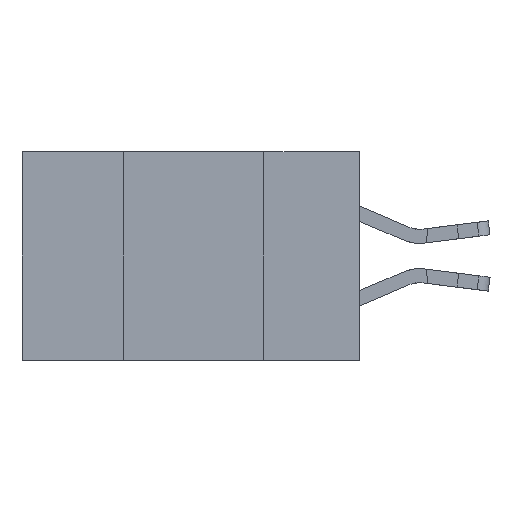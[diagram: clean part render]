
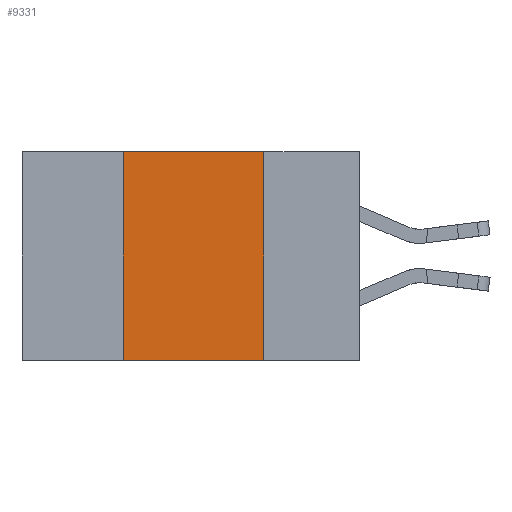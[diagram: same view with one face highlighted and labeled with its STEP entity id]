
A CAD part, left-side view. The second image highlights one B-rep face of the part: STEP entity #9331.
In plain terms, the highlighted planar face has unit normal (-1, 0, 0).
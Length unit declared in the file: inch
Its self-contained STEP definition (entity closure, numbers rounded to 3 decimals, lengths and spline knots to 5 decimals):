
#10 = LINE ( 'NONE', #21667, #20473 ) ;
#77 = ORIENTED_EDGE ( 'NONE', *, *, #8759, .F. ) ;
#528 = DIRECTION ( 'NONE',  ( 0., -1., 0. ) ) ;
#727 = VECTOR ( 'NONE', #10962, 39.37008 ) ;
#1062 = EDGE_CURVE ( 'NONE', #15115, #17865, #5064, .T. ) ;
#2873 = FACE_OUTER_BOUND ( 'NONE', #7332, .T. ) ;
#3365 = EDGE_CURVE ( 'NONE', #15115, #3771, #10, .T. ) ;
#3537 = LINE ( 'NONE', #15646, #3848 ) ;
#3771 = VERTEX_POINT ( 'NONE', #7977 ) ;
#3848 = VECTOR ( 'NONE', #25251, 39.37008 ) ;
#3983 = DIRECTION ( 'NONE',  ( 0., 0., 1. ) ) ;
#5064 = LINE ( 'NONE', #12418, #20917 ) ;
#7332 = EDGE_LOOP ( 'NONE', ( #77, #22812, #19402, #14520 ) ) ;
#7977 = CARTESIAN_POINT ( 'NONE',  ( 0., 0.42, 0. ) ) ;
#8481 = DIRECTION ( 'NONE',  ( 0., 0., -1. ) ) ;
#8759 = EDGE_CURVE ( 'NONE', #22135, #17865, #14684, .T. ) ;
#9331 = ADVANCED_FACE ( 'NONE', ( #2873 ), #16582, .F. ) ;
#10962 = DIRECTION ( 'NONE',  ( 0., 0., -1. ) ) ;
#12418 = CARTESIAN_POINT ( 'NONE',  ( 0., 0.6, -0.37 ) ) ;
#13115 = EDGE_CURVE ( 'NONE', #3771, #22135, #3537, .T. ) ;
#14520 = ORIENTED_EDGE ( 'NONE', *, *, #1062, .T. ) ;
#14684 = LINE ( 'NONE', #22830, #727 ) ;
#15115 = VERTEX_POINT ( 'NONE', #15662 ) ;
#15646 = CARTESIAN_POINT ( 'NONE',  ( 0., 0.6, 0. ) ) ;
#15662 = CARTESIAN_POINT ( 'NONE',  ( 0., 0.42, -0.37 ) ) ;
#16406 = DIRECTION ( 'NONE',  ( 1., 0., 0. ) ) ;
#16582 = PLANE ( 'NONE',  #23406 ) ;
#17865 = VERTEX_POINT ( 'NONE', #25488 ) ;
#19402 = ORIENTED_EDGE ( 'NONE', *, *, #3365, .F. ) ;
#20473 = VECTOR ( 'NONE', #3983, 39.37008 ) ;
#20917 = VECTOR ( 'NONE', #528, 39.37008 ) ;
#21667 = CARTESIAN_POINT ( 'NONE',  ( 0., 0.42, 0. ) ) ;
#22135 = VERTEX_POINT ( 'NONE', #25211 ) ;
#22436 = CARTESIAN_POINT ( 'NONE',  ( 0., 0.6, 0. ) ) ;
#22812 = ORIENTED_EDGE ( 'NONE', *, *, #13115, .F. ) ;
#22830 = CARTESIAN_POINT ( 'NONE',  ( 0., 0.17, 0. ) ) ;
#23406 = AXIS2_PLACEMENT_3D ( 'NONE', #22436, #16406, #8481 ) ;
#25211 = CARTESIAN_POINT ( 'NONE',  ( 0., 0.17, 0. ) ) ;
#25251 = DIRECTION ( 'NONE',  ( 0., -1., 0. ) ) ;
#25488 = CARTESIAN_POINT ( 'NONE',  ( 0., 0.17, -0.37 ) ) ;
